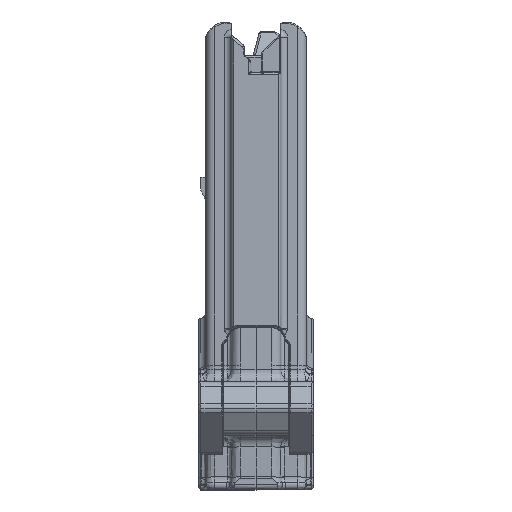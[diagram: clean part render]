
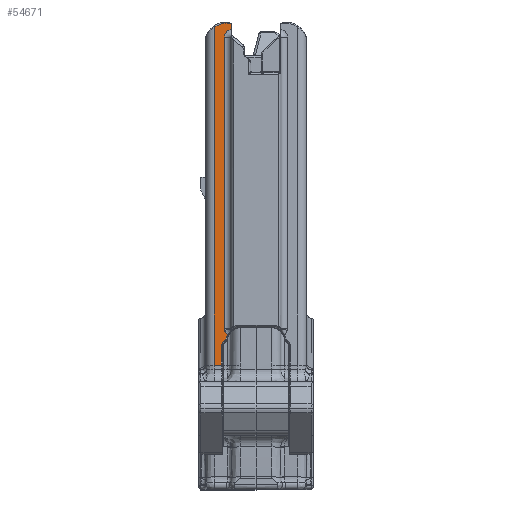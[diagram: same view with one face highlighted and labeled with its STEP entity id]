
A CAD part, top view. The second image highlights one B-rep face of the part: STEP entity #54671.
In plain terms, the highlighted planar face has unit normal (0, 0, 1).
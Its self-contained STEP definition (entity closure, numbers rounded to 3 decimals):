
#57 = CARTESIAN_POINT ( 'NONE',  ( -6.299, 76.023, 30.353 ) ) ;
#919 = EDGE_CURVE ( 'NONE', #20968, #55625, #22319, .T. ) ;
#921 = LINE ( 'NONE', #22091, #47665 ) ;
#2465 = EDGE_CURVE ( 'NONE', #65594, #34383, #44366, .T. ) ;
#2498 = ORIENTED_EDGE ( 'NONE', *, *, #56876, .T. ) ;
#4143 = VERTEX_POINT ( 'NONE', #25179 ) ;
#4337 = CARTESIAN_POINT ( 'NONE',  ( -6.972, 7.733, 30.353 ) ) ;
#4349 = DIRECTION ( 'NONE',  ( 1., 0., 0. ) ) ;
#4735 = ORIENTED_EDGE ( 'NONE', *, *, #45051, .T. ) ;
#4964 = DIRECTION ( 'NONE',  ( -1., 0., 0. ) ) ;
#4972 = CARTESIAN_POINT ( 'NONE',  ( -6.972, 7.733, 30.353 ) ) ;
#5649 = PLANE ( 'NONE',  #21783 ) ;
#6317 = CARTESIAN_POINT ( 'NONE',  ( -5.77, 75.974, 30.353 ) ) ;
#6836 = ORIENTED_EDGE ( 'NONE', *, *, #8351, .T. ) ;
#6908 = B_SPLINE_CURVE_WITH_KNOTS ( 'NONE', 3,
 ( #21260, #32035, #47356, #16382, #6317, #48724 ),
 .UNSPECIFIED., .F., .F.,
 ( 4, 2, 4 ),
 ( 0., 0.5, 1. ),
 .UNSPECIFIED. ) ;
#8351 = EDGE_CURVE ( 'NONE', #25695, #19335, #22415, .T. ) ;
#8437 = AXIS2_PLACEMENT_3D ( 'NONE', #14346, #42181, #25490 ) ;
#9850 = CARTESIAN_POINT ( 'NONE',  ( -6.888, 7.342, 30.353 ) ) ;
#10482 = ORIENTED_EDGE ( 'NONE', *, *, #2465, .F. ) ;
#10528 = ORIENTED_EDGE ( 'NONE', *, *, #53056, .T. ) ;
#10812 = VECTOR ( 'NONE', #30450, 1000. ) ;
#11015 = ORIENTED_EDGE ( 'NONE', *, *, #46836, .F. ) ;
#11200 = DIRECTION ( 'NONE',  ( -1., 0., 0. ) ) ;
#12124 = DIRECTION ( 'NONE',  ( 0., 0., -1. ) ) ;
#12739 = LINE ( 'NONE', #29075, #24154 ) ;
#14053 = B_SPLINE_CURVE_WITH_KNOTS ( 'NONE', 3,
 ( #36613, #46713, #9850, #4972 ),
 .UNSPECIFIED., .F., .F.,
 ( 4, 4 ),
 ( 0., 1. ),
 .UNSPECIFIED. ) ;
#14173 = ORIENTED_EDGE ( 'NONE', *, *, #919, .F. ) ;
#14346 = CARTESIAN_POINT ( 'NONE',  ( -3.325, 5.339, 30.353 ) ) ;
#14439 = AXIS2_PLACEMENT_3D ( 'NONE', #59474, #12124, #32988 ) ;
#14717 = ORIENTED_EDGE ( 'NONE', *, *, #68215, .F. ) ;
#14774 = CARTESIAN_POINT ( 'NONE',  ( -9.271, 75.614, 30.353 ) ) ;
#15611 = VERTEX_POINT ( 'NONE', #31333 ) ;
#15726 = CARTESIAN_POINT ( 'NONE',  ( -9.271, 0., 30.353 ) ) ;
#15763 = LINE ( 'NONE', #62804, #25535 ) ;
#16083 = CARTESIAN_POINT ( 'NONE',  ( -5.512, 75.882, 30.353 ) ) ;
#16277 = ORIENTED_EDGE ( 'NONE', *, *, #52961, .T. ) ;
#16382 = CARTESIAN_POINT ( 'NONE',  ( -5.728, 75.937, 30.353 ) ) ;
#16502 = DIRECTION ( 'NONE',  ( 0., 0., 1. ) ) ;
#17551 = CARTESIAN_POINT ( 'NONE',  ( -6.929, 5.722, 30.353 ) ) ;
#18054 = CARTESIAN_POINT ( 'NONE',  ( -7.7, 4.214, 30.353 ) ) ;
#18891 = CARTESIAN_POINT ( 'NONE',  ( -5.262, 8.102, 30.353 ) ) ;
#19335 = VERTEX_POINT ( 'NONE', #41548 ) ;
#20968 = VERTEX_POINT ( 'NONE', #50078 ) ;
#21260 = CARTESIAN_POINT ( 'NONE',  ( -5.512, 75.882, 30.353 ) ) ;
#21753 = DIRECTION ( 'NONE',  ( 0., -1., 0. ) ) ;
#21783 = AXIS2_PLACEMENT_3D ( 'NONE', #22898, #33336, #4964 ) ;
#22091 = CARTESIAN_POINT ( 'NONE',  ( -5.512, 0., 30.353 ) ) ;
#22319 = LINE ( 'NONE', #52996, #27294 ) ;
#22415 = CIRCLE ( 'NONE', #54699, 1.75 ) ;
#22898 = CARTESIAN_POINT ( 'NONE',  ( -6.299, 0., 30.353 ) ) ;
#23240 = ORIENTED_EDGE ( 'NONE', *, *, #61280, .F. ) ;
#23439 = CARTESIAN_POINT ( 'NONE',  ( -7.012, 72.952, 30.353 ) ) ;
#23674 = CIRCLE ( 'NONE', #35891, 0.25 ) ;
#24154 = VECTOR ( 'NONE', #33947, 1000. ) ;
#24708 = VERTEX_POINT ( 'NONE', #16083 ) ;
#25179 = CARTESIAN_POINT ( 'NONE',  ( -6.385, 6.761, 30.353 ) ) ;
#25490 = DIRECTION ( 'NONE',  ( -1., 0., 0. ) ) ;
#25535 = VECTOR ( 'NONE', #4349, 1000. ) ;
#25582 = CARTESIAN_POINT ( 'NONE',  ( -5.512, 74.685, 30.353 ) ) ;
#25695 = VERTEX_POINT ( 'NONE', #4337 ) ;
#27294 = VECTOR ( 'NONE', #53335, 1000. ) ;
#27856 = EDGE_CURVE ( 'NONE', #56135, #15611, #63352, .T. ) ;
#27972 = DIRECTION ( 'NONE',  ( -1., 0., 0. ) ) ;
#28344 = EDGE_CURVE ( 'NONE', #43768, #53772, #33357, .T. ) ;
#29075 = CARTESIAN_POINT ( 'NONE',  ( -7.7, 4.214, 30.353 ) ) ;
#29970 = VERTEX_POINT ( 'NONE', #36959 ) ;
#30450 = DIRECTION ( 'NONE',  ( 0., 1., 0. ) ) ;
#30882 = EDGE_CURVE ( 'NONE', #15611, #29970, #23674, .T. ) ;
#31333 = CARTESIAN_POINT ( 'NONE',  ( -6.836, 5.49, 30.353 ) ) ;
#32035 = CARTESIAN_POINT ( 'NONE',  ( -5.57, 75.877, 30.353 ) ) ;
#32988 = DIRECTION ( 'NONE',  ( -1., 0., 0. ) ) ;
#33305 = AXIS2_PLACEMENT_3D ( 'NONE', #68620, #57865, #11200 ) ;
#33336 = DIRECTION ( 'NONE',  ( 0., 0., -1. ) ) ;
#33357 = CIRCLE ( 'NONE', #33305, 1.75 ) ;
#33617 = CARTESIAN_POINT ( 'NONE',  ( -9.271, 75.163, 30.353 ) ) ;
#33815 = CARTESIAN_POINT ( 'NONE',  ( -5.801, 76.023, 30.353 ) ) ;
#33947 = DIRECTION ( 'NONE',  ( 0., 1., 0. ) ) ;
#34383 = VERTEX_POINT ( 'NONE', #41012 ) ;
#35363 = VECTOR ( 'NONE', #61236, 1000. ) ;
#35891 = AXIS2_PLACEMENT_3D ( 'NONE', #17551, #16502, #27972 ) ;
#36613 = CARTESIAN_POINT ( 'NONE',  ( -6.385, 6.761, 30.353 ) ) ;
#36959 = CARTESIAN_POINT ( 'NONE',  ( -6.681, 5.696, 30.353 ) ) ;
#41012 = CARTESIAN_POINT ( 'NONE',  ( -6.299, 76.023, 30.353 ) ) ;
#41548 = CARTESIAN_POINT ( 'NONE',  ( -7.012, 8.102, 30.353 ) ) ;
#41757 = VERTEX_POINT ( 'NONE', #33815 ) ;
#42181 = DIRECTION ( 'NONE',  ( 0., 0., -1. ) ) ;
#43768 = VERTEX_POINT ( 'NONE', #23439 ) ;
#44366 =( BOUNDED_CURVE ( )  B_SPLINE_CURVE ( 3, ( #58146, #63708, #52922, #57 ),
 .UNSPECIFIED., .F., .F. ) 
 B_SPLINE_CURVE_WITH_KNOTS ( ( 4, 4 ),
 ( 0., 1. ),
 .UNSPECIFIED. ) 
 CURVE ( )  GEOMETRIC_REPRESENTATION_ITEM ( )  RATIONAL_B_SPLINE_CURVE ( ( 1., 0.959, 0.959, 1. ) ) 
 REPRESENTATION_ITEM ( '' )  );
#44938 = ORIENTED_EDGE ( 'NONE', *, *, #46707, .T. ) ;
#45051 = EDGE_CURVE ( 'NONE', #24708, #41757, #6908, .T. ) ;
#45668 = DIRECTION ( 'NONE',  ( -1., 0., 0. ) ) ;
#46707 = EDGE_CURVE ( 'NONE', #20968, #56135, #12739, .T. ) ;
#46713 = CARTESIAN_POINT ( 'NONE',  ( -6.692, 7.018, 30.353 ) ) ;
#46836 = EDGE_CURVE ( 'NONE', #55625, #65594, #56918, .T. ) ;
#47184 = ORIENTED_EDGE ( 'NONE', *, *, #27856, .T. ) ;
#47356 = CARTESIAN_POINT ( 'NONE',  ( -5.624, 75.886, 30.353 ) ) ;
#47665 = VECTOR ( 'NONE', #21753, 1000. ) ;
#48724 = CARTESIAN_POINT ( 'NONE',  ( -5.801, 76.023, 30.353 ) ) ;
#50078 = CARTESIAN_POINT ( 'NONE',  ( -7.7, 0., 30.353 ) ) ;
#52618 = FACE_OUTER_BOUND ( 'NONE', #54295, .T. ) ;
#52922 = CARTESIAN_POINT ( 'NONE',  ( -7.372, 76.1, 30.353 ) ) ;
#52961 = EDGE_CURVE ( 'NONE', #4143, #25695, #14053, .T. ) ;
#52996 = CARTESIAN_POINT ( 'NONE',  ( -6.325, 0., 30.353 ) ) ;
#53056 = EDGE_CURVE ( 'NONE', #29970, #4143, #56209, .T. ) ;
#53335 = DIRECTION ( 'NONE',  ( -1., 0., 0. ) ) ;
#53772 = VERTEX_POINT ( 'NONE', #25582 ) ;
#54295 = EDGE_LOOP ( 'NONE', ( #2498, #58693, #14717, #4735, #23240, #10482, #11015, #14173, #44938, #47184, #65861, #10528, #16277, #6836 ) ) ;
#54671 = ADVANCED_FACE ( 'NONE', ( #52618 ), #5649, .F. ) ;
#54699 = AXIS2_PLACEMENT_3D ( 'NONE', #18891, #65874, #45668 ) ;
#55625 = VERTEX_POINT ( 'NONE', #15726 ) ;
#55666 = CARTESIAN_POINT ( 'NONE',  ( -7.012, 72.952, 30.353 ) ) ;
#56002 = LINE ( 'NONE', #55666, #35363 ) ;
#56135 = VERTEX_POINT ( 'NONE', #18054 ) ;
#56209 = CIRCLE ( 'NONE', #8437, 3.375 ) ;
#56876 = EDGE_CURVE ( 'NONE', #19335, #43768, #56002, .T. ) ;
#56918 = LINE ( 'NONE', #14774, #10812 ) ;
#57865 = DIRECTION ( 'NONE',  ( 0., 0., -1. ) ) ;
#58146 = CARTESIAN_POINT ( 'NONE',  ( -9.271, 75.163, 30.353 ) ) ;
#58693 = ORIENTED_EDGE ( 'NONE', *, *, #28344, .T. ) ;
#59474 = CARTESIAN_POINT ( 'NONE',  ( -6.325, 4.214, 30.353 ) ) ;
#61236 = DIRECTION ( 'NONE',  ( 0., 1., 0. ) ) ;
#61280 = EDGE_CURVE ( 'NONE', #34383, #41757, #15763, .T. ) ;
#62804 = CARTESIAN_POINT ( 'NONE',  ( -6.299, 76.023, 30.353 ) ) ;
#63352 = CIRCLE ( 'NONE', #14439, 1.375 ) ;
#63708 = CARTESIAN_POINT ( 'NONE',  ( -8.405, 75.801, 30.353 ) ) ;
#65594 = VERTEX_POINT ( 'NONE', #33617 ) ;
#65861 = ORIENTED_EDGE ( 'NONE', *, *, #30882, .T. ) ;
#65874 = DIRECTION ( 'NONE',  ( 0., 0., -1. ) ) ;
#68215 = EDGE_CURVE ( 'NONE', #24708, #53772, #921, .T. ) ;
#68620 = CARTESIAN_POINT ( 'NONE',  ( -5.262, 72.952, 30.353 ) ) ;
